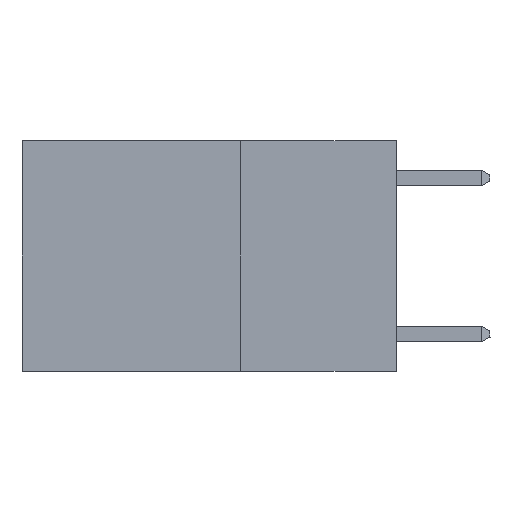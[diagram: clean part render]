
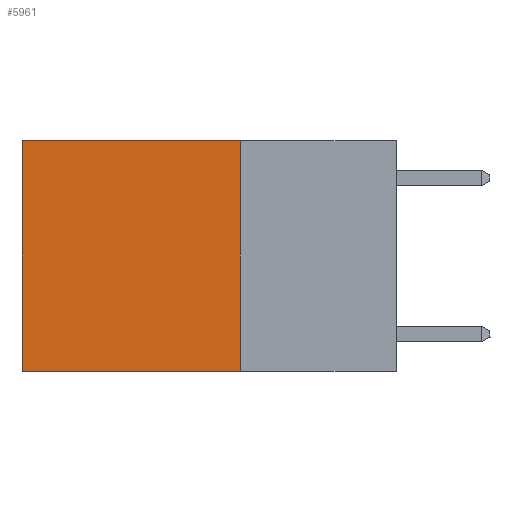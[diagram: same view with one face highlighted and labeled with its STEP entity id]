
A CAD part, left-side view. The second image highlights one B-rep face of the part: STEP entity #5961.
In plain terms, the highlighted planar face has unit normal (-1, 0, 0).
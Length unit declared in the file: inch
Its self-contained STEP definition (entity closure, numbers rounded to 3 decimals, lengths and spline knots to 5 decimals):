
#607 = VERTEX_POINT ( 'NONE', #12587 ) ;
#1233 = CARTESIAN_POINT ( 'NONE',  ( 0.2625, 0.6, 0. ) ) ;
#1368 = AXIS2_PLACEMENT_3D ( 'NONE', #19400, #3622, #12819 ) ;
#2711 = VECTOR ( 'NONE', #19646, 39.37008 ) ;
#2722 = LINE ( 'NONE', #16861, #2711 ) ;
#2985 = EDGE_CURVE ( 'NONE', #19580, #3337, #14417, .T. ) ;
#3337 = VERTEX_POINT ( 'NONE', #16985 ) ;
#3622 = DIRECTION ( 'NONE',  ( 1., 0., 0. ) ) ;
#3665 = EDGE_CURVE ( 'NONE', #18971, #19580, #14812, .T. ) ;
#3800 = EDGE_CURVE ( 'NONE', #18971, #607, #2722, .T. ) ;
#4822 = EDGE_CURVE ( 'NONE', #607, #3337, #9443, .T. ) ;
#4995 = ORIENTED_EDGE ( 'NONE', *, *, #3800, .F. ) ;
#5107 = DIRECTION ( 'NONE',  ( 0., 1., 0. ) ) ;
#5961 = ADVANCED_FACE ( 'NONE', ( #13127 ), #14556, .F. ) ;
#6009 = VECTOR ( 'NONE', #5107, 39.37008 ) ;
#6474 = DIRECTION ( 'NONE',  ( 0., 1., 0. ) ) ;
#6666 = CARTESIAN_POINT ( 'NONE',  ( 0.2625, 0.25, 0. ) ) ;
#7761 = ORIENTED_EDGE ( 'NONE', *, *, #3665, .T. ) ;
#9443 = LINE ( 'NONE', #11510, #15625 ) ;
#11338 = DIRECTION ( 'NONE',  ( 0., 0., -1. ) ) ;
#11510 = CARTESIAN_POINT ( 'NONE',  ( 0.2625, 0.25, -0.37 ) ) ;
#12587 = CARTESIAN_POINT ( 'NONE',  ( 0.2625, 0.25, -0.37 ) ) ;
#12819 = DIRECTION ( 'NONE',  ( 0., 0., -1. ) ) ;
#13127 = FACE_OUTER_BOUND ( 'NONE', #19779, .T. ) ;
#13703 = ORIENTED_EDGE ( 'NONE', *, *, #4822, .F. ) ;
#14417 = LINE ( 'NONE', #19155, #19981 ) ;
#14556 = PLANE ( 'NONE',  #1368 ) ;
#14812 = LINE ( 'NONE', #6666, #6009 ) ;
#15625 = VECTOR ( 'NONE', #6474, 39.37008 ) ;
#16861 = CARTESIAN_POINT ( 'NONE',  ( 0.2625, 0.25, 0. ) ) ;
#16985 = CARTESIAN_POINT ( 'NONE',  ( 0.2625, 0.6, -0.37 ) ) ;
#18971 = VERTEX_POINT ( 'NONE', #19145 ) ;
#19145 = CARTESIAN_POINT ( 'NONE',  ( 0.2625, 0.25, 0. ) ) ;
#19155 = CARTESIAN_POINT ( 'NONE',  ( 0.2625, 0.6, 0. ) ) ;
#19163 = ORIENTED_EDGE ( 'NONE', *, *, #2985, .T. ) ;
#19400 = CARTESIAN_POINT ( 'NONE',  ( 0.2625, 0.25, 0. ) ) ;
#19580 = VERTEX_POINT ( 'NONE', #1233 ) ;
#19646 = DIRECTION ( 'NONE',  ( 0., 0., -1. ) ) ;
#19779 = EDGE_LOOP ( 'NONE', ( #19163, #13703, #4995, #7761 ) ) ;
#19981 = VECTOR ( 'NONE', #11338, 39.37008 ) ;
